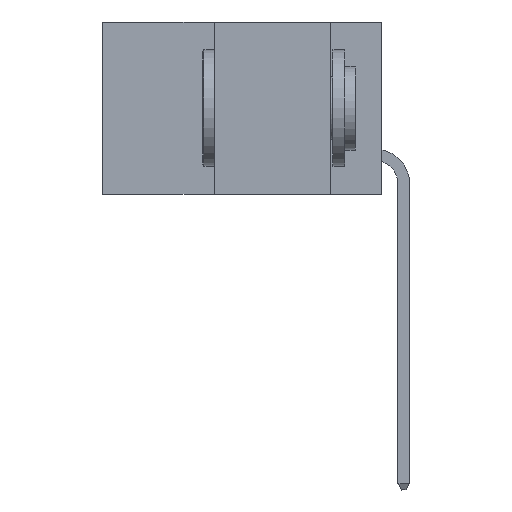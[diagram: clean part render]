
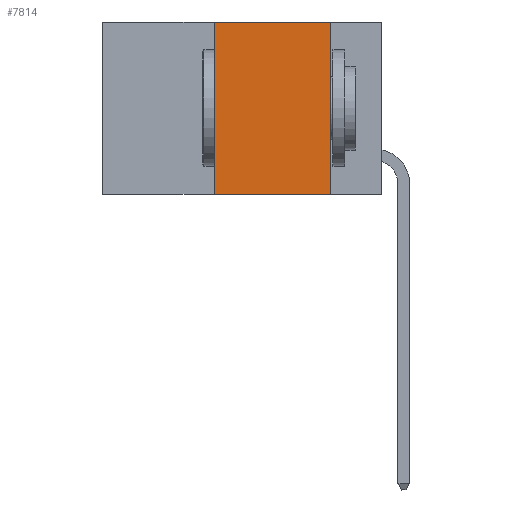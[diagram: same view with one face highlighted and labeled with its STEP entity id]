
A CAD part, left-side view. The second image highlights one B-rep face of the part: STEP entity #7814.
In plain terms, the highlighted planar face has unit normal (-1, 0, 0).
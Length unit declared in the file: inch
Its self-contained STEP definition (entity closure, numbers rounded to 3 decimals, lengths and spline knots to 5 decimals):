
#337 = VERTEX_POINT ( 'NONE', #22101 ) ;
#603 = EDGE_CURVE ( 'NONE', #1809, #5274, #19834, .T. ) ;
#1809 = VERTEX_POINT ( 'NONE', #16745 ) ;
#2558 = DIRECTION ( 'NONE',  ( 0., 0., -1. ) ) ;
#3899 = LINE ( 'NONE', #10675, #35920 ) ;
#4976 = DIRECTION ( 'NONE',  ( 0., 0., 1. ) ) ;
#5274 = VERTEX_POINT ( 'NONE', #5645 ) ;
#5388 = LINE ( 'NONE', #34109, #26249 ) ;
#5645 = CARTESIAN_POINT ( 'NONE',  ( 0., 0.11, 0. ) ) ;
#7406 = ORIENTED_EDGE ( 'NONE', *, *, #603, .F. ) ;
#7814 = ADVANCED_FACE ( 'NONE', ( #9700 ), #19073, .F. ) ;
#9094 = DIRECTION ( 'NONE',  ( 0., -1., 0. ) ) ;
#9700 = FACE_OUTER_BOUND ( 'NONE', #34084, .T. ) ;
#10675 = CARTESIAN_POINT ( 'NONE',  ( 0., 0.6, -0.37 ) ) ;
#10755 = VECTOR ( 'NONE', #4976, 39.37008 ) ;
#11336 = VECTOR ( 'NONE', #9094, 39.37008 ) ;
#12460 = VERTEX_POINT ( 'NONE', #19134 ) ;
#13050 = DIRECTION ( 'NONE',  ( 0., -1., 0. ) ) ;
#15255 = EDGE_CURVE ( 'NONE', #12460, #337, #3899, .T. ) ;
#16745 = CARTESIAN_POINT ( 'NONE',  ( 0., 0.36, 0. ) ) ;
#19073 = PLANE ( 'NONE',  #32812 ) ;
#19134 = CARTESIAN_POINT ( 'NONE',  ( 0., 0.36, -0.37 ) ) ;
#19834 = LINE ( 'NONE', #28740, #11336 ) ;
#21931 = DIRECTION ( 'NONE',  ( 1., 0., 0. ) ) ;
#21940 = ORIENTED_EDGE ( 'NONE', *, *, #15255, .T. ) ;
#22041 = CARTESIAN_POINT ( 'NONE',  ( 0., 0.36, 0. ) ) ;
#22101 = CARTESIAN_POINT ( 'NONE',  ( 0., 0.11, -0.37 ) ) ;
#24653 = CARTESIAN_POINT ( 'NONE',  ( 0., 0.6, 0. ) ) ;
#24894 = DIRECTION ( 'NONE',  ( 0., 0., -1. ) ) ;
#26216 = EDGE_CURVE ( 'NONE', #5274, #337, #5388, .T. ) ;
#26249 = VECTOR ( 'NONE', #2558, 39.37008 ) ;
#26287 = LINE ( 'NONE', #22041, #10755 ) ;
#27015 = ORIENTED_EDGE ( 'NONE', *, *, #26216, .F. ) ;
#27830 = ORIENTED_EDGE ( 'NONE', *, *, #34207, .F. ) ;
#28740 = CARTESIAN_POINT ( 'NONE',  ( 0., 0.6, 0. ) ) ;
#32812 = AXIS2_PLACEMENT_3D ( 'NONE', #24653, #21931, #24894 ) ;
#34084 = EDGE_LOOP ( 'NONE', ( #27015, #7406, #27830, #21940 ) ) ;
#34109 = CARTESIAN_POINT ( 'NONE',  ( 0., 0.11, 0. ) ) ;
#34207 = EDGE_CURVE ( 'NONE', #12460, #1809, #26287, .T. ) ;
#35920 = VECTOR ( 'NONE', #13050, 39.37008 ) ;
